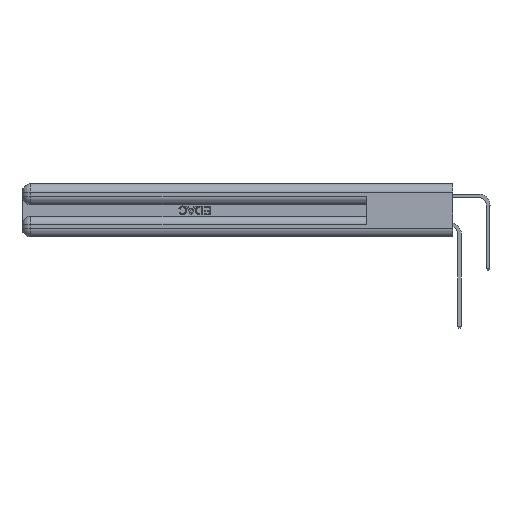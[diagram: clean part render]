
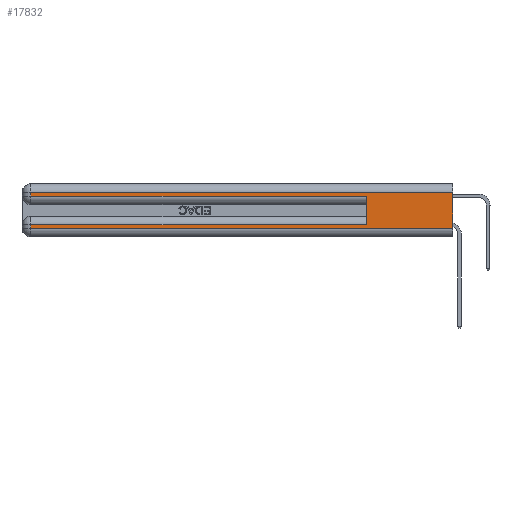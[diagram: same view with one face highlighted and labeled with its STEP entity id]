
A CAD part, left-side view. The second image highlights one B-rep face of the part: STEP entity #17832.
In plain terms, the highlighted planar face has unit normal (-1, 0, 0).
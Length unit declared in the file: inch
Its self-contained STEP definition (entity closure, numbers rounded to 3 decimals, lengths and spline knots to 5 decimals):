
#871 = ORIENTED_EDGE ( 'NONE', *, *, #2676, .T. ) ;
#1051 = DIRECTION ( 'NONE',  ( 1., 0., 0. ) ) ;
#1415 = DIRECTION ( 'NONE',  ( 0., 0., -1. ) ) ;
#1748 = CARTESIAN_POINT ( 'NONE',  ( 0., 0., 0.31 ) ) ;
#2026 = EDGE_CURVE ( 'NONE', #6814, #30521, #34647, .T. ) ;
#2676 = EDGE_CURVE ( 'NONE', #6814, #9357, #2888, .T. ) ;
#2888 = LINE ( 'NONE', #38211, #20542 ) ;
#4227 = LINE ( 'NONE', #13816, #12045 ) ;
#4935 = DIRECTION ( 'NONE',  ( 0., -1., 0. ) ) ;
#6277 = ORIENTED_EDGE ( 'NONE', *, *, #21825, .F. ) ;
#6403 = EDGE_CURVE ( 'NONE', #9357, #18249, #4227, .T. ) ;
#6479 = VERTEX_POINT ( 'NONE', #14106 ) ;
#6814 = VERTEX_POINT ( 'NONE', #12648 ) ;
#9357 = VERTEX_POINT ( 'NONE', #10618 ) ;
#10266 = DIRECTION ( 'NONE',  ( 0., -1., 0. ) ) ;
#10449 = DIRECTION ( 'NONE',  ( 0., 0., 1. ) ) ;
#10452 = VECTOR ( 'NONE', #10266, 39.37008 ) ;
#10618 = CARTESIAN_POINT ( 'NONE',  ( 0., 2.94, 0.085 ) ) ;
#12045 = VECTOR ( 'NONE', #37068, 39.37008 ) ;
#12648 = CARTESIAN_POINT ( 'NONE',  ( 0., 0.6, 0.085 ) ) ;
#13816 = CARTESIAN_POINT ( 'NONE',  ( 0., 2.94, 0.37 ) ) ;
#14106 = CARTESIAN_POINT ( 'NONE',  ( 0., 0., 0.31 ) ) ;
#14270 = EDGE_LOOP ( 'NONE', ( #6277, #26274, #38952, #36345, #27957, #871, #20101, #17954 ) ) ;
#14654 = CARTESIAN_POINT ( 'NONE',  ( 0., 0., 0.06 ) ) ;
#14830 = VERTEX_POINT ( 'NONE', #36392 ) ;
#14926 = VERTEX_POINT ( 'NONE', #20517 ) ;
#15655 = LINE ( 'NONE', #42402, #34388 ) ;
#16792 = AXIS2_PLACEMENT_3D ( 'NONE', #20956, #1051, #24286 ) ;
#17832 = ADVANCED_FACE ( 'NONE', ( #24402 ), #24143, .F. ) ;
#17954 = ORIENTED_EDGE ( 'NONE', *, *, #41223, .T. ) ;
#18249 = VERTEX_POINT ( 'NONE', #23553 ) ;
#19160 = VERTEX_POINT ( 'NONE', #14654 ) ;
#19173 = DIRECTION ( 'NONE',  ( 0., 0., -1. ) ) ;
#19228 = EDGE_CURVE ( 'NONE', #14926, #30521, #22177, .T. ) ;
#19248 = LINE ( 'NONE', #36791, #10452 ) ;
#20101 = ORIENTED_EDGE ( 'NONE', *, *, #6403, .T. ) ;
#20517 = CARTESIAN_POINT ( 'NONE',  ( 0., 2.94, 0.285 ) ) ;
#20542 = VECTOR ( 'NONE', #28189, 39.37008 ) ;
#20956 = CARTESIAN_POINT ( 'NONE',  ( 0., 0., 0.37 ) ) ;
#21825 = EDGE_CURVE ( 'NONE', #6479, #19160, #40094, .T. ) ;
#22177 = LINE ( 'NONE', #34682, #38815 ) ;
#23030 = EDGE_CURVE ( 'NONE', #14830, #14926, #15655, .T. ) ;
#23553 = CARTESIAN_POINT ( 'NONE',  ( 0., 2.94, 0.06 ) ) ;
#24143 = PLANE ( 'NONE',  #16792 ) ;
#24286 = DIRECTION ( 'NONE',  ( 0., 0., -1. ) ) ;
#24402 = FACE_OUTER_BOUND ( 'NONE', #14270, .T. ) ;
#24975 = DIRECTION ( 'NONE',  ( 0., 1., 0. ) ) ;
#26274 = ORIENTED_EDGE ( 'NONE', *, *, #37415, .T. ) ;
#26829 = VECTOR ( 'NONE', #10449, 39.37008 ) ;
#27957 = ORIENTED_EDGE ( 'NONE', *, *, #2026, .F. ) ;
#28027 = CARTESIAN_POINT ( 'NONE',  ( 0., 0., 0.37 ) ) ;
#28189 = DIRECTION ( 'NONE',  ( 0., 1., 0. ) ) ;
#30521 = VERTEX_POINT ( 'NONE', #33509 ) ;
#31312 = VECTOR ( 'NONE', #1415, 39.37008 ) ;
#32430 = VECTOR ( 'NONE', #24975, 39.37008 ) ;
#33466 = LINE ( 'NONE', #1748, #32430 ) ;
#33509 = CARTESIAN_POINT ( 'NONE',  ( 0., 0.6, 0.285 ) ) ;
#34388 = VECTOR ( 'NONE', #19173, 39.37008 ) ;
#34647 = LINE ( 'NONE', #40278, #26829 ) ;
#34682 = CARTESIAN_POINT ( 'NONE',  ( 0., 0., 0.285 ) ) ;
#36345 = ORIENTED_EDGE ( 'NONE', *, *, #19228, .T. ) ;
#36392 = CARTESIAN_POINT ( 'NONE',  ( 0., 2.94, 0.31 ) ) ;
#36791 = CARTESIAN_POINT ( 'NONE',  ( 0., 0., 0.06 ) ) ;
#37068 = DIRECTION ( 'NONE',  ( 0., 0., -1. ) ) ;
#37415 = EDGE_CURVE ( 'NONE', #6479, #14830, #33466, .T. ) ;
#38211 = CARTESIAN_POINT ( 'NONE',  ( 0., 0., 0.085 ) ) ;
#38815 = VECTOR ( 'NONE', #4935, 39.37008 ) ;
#38952 = ORIENTED_EDGE ( 'NONE', *, *, #23030, .T. ) ;
#40094 = LINE ( 'NONE', #28027, #31312 ) ;
#40278 = CARTESIAN_POINT ( 'NONE',  ( 0., 0.6, 0.145 ) ) ;
#41223 = EDGE_CURVE ( 'NONE', #18249, #19160, #19248, .T. ) ;
#42402 = CARTESIAN_POINT ( 'NONE',  ( 0., 2.94, 0.37 ) ) ;
